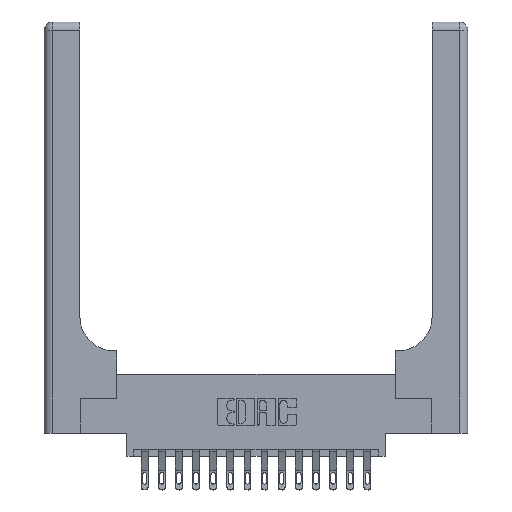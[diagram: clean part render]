
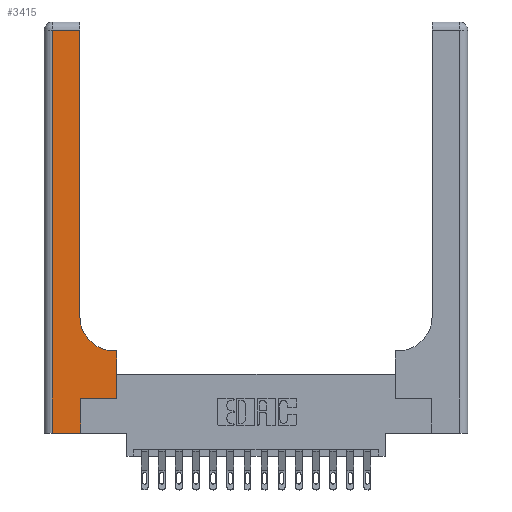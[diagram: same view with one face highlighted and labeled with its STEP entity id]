
A CAD part, top view. The second image highlights one B-rep face of the part: STEP entity #3415.
In plain terms, the highlighted planar face has unit normal (0, 0, 1).
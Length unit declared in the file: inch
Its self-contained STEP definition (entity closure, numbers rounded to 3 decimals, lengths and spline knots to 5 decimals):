
#229 = EDGE_CURVE ( 'NONE', #543, #14760, #238, .T. ) ;
#238 = LINE ( 'NONE', #16307, #10836 ) ;
#288 = VECTOR ( 'NONE', #13232, 39.37008 ) ;
#355 = ORIENTED_EDGE ( 'NONE', *, *, #1144, .T. ) ;
#386 = LINE ( 'NONE', #7572, #288 ) ;
#531 = VERTEX_POINT ( 'NONE', #16461 ) ;
#543 = VERTEX_POINT ( 'NONE', #9595 ) ;
#1144 = EDGE_CURVE ( 'NONE', #12660, #7336, #11203, .T. ) ;
#1332 = CARTESIAN_POINT ( 'NONE',  ( 0.26, 0.85, 0.37 ) ) ;
#1603 = CARTESIAN_POINT ( 'NONE',  ( 0.528, 0.25, 0.37 ) ) ;
#2816 = CARTESIAN_POINT ( 'NONE',  ( 0.265, 0.25, 0.37 ) ) ;
#2818 = EDGE_CURVE ( 'NONE', #3894, #8827, #14255, .T. ) ;
#3065 = LINE ( 'NONE', #7341, #10502 ) ;
#3185 = VERTEX_POINT ( 'NONE', #13053 ) ;
#3236 = DIRECTION ( 'NONE',  ( 0., 1., 0. ) ) ;
#3415 = ADVANCED_FACE ( 'NONE', ( #12755 ), #17022, .F. ) ;
#3499 = CARTESIAN_POINT ( 'NONE',  ( 0.51, 0.85, 0.37 ) ) ;
#3774 = CARTESIAN_POINT ( 'NONE',  ( 0.26, 2.94, 0.37 ) ) ;
#3894 = VERTEX_POINT ( 'NONE', #2816 ) ;
#3938 = VECTOR ( 'NONE', #3236, 39.37008 ) ;
#4276 = ORIENTED_EDGE ( 'NONE', *, *, #11845, .T. ) ;
#4566 = LINE ( 'NONE', #7573, #14867 ) ;
#4765 = DIRECTION ( 'NONE',  ( 0., 0., -1. ) ) ;
#5397 = EDGE_CURVE ( 'NONE', #14760, #531, #386, .T. ) ;
#5924 = ORIENTED_EDGE ( 'NONE', *, *, #5397, .T. ) ;
#5992 = AXIS2_PLACEMENT_3D ( 'NONE', #3499, #4765, #9407 ) ;
#6170 = ORIENTED_EDGE ( 'NONE', *, *, #11060, .T. ) ;
#6797 = EDGE_CURVE ( 'NONE', #7336, #9367, #3065, .T. ) ;
#6962 = CARTESIAN_POINT ( 'NONE',  ( 0.265, 0.25, 0.37 ) ) ;
#7336 = VERTEX_POINT ( 'NONE', #1332 ) ;
#7341 = CARTESIAN_POINT ( 'NONE',  ( 0.26, 3., 0.37 ) ) ;
#7572 = CARTESIAN_POINT ( 'NONE',  ( 0., 0., 0.37 ) ) ;
#7573 = CARTESIAN_POINT ( 'NONE',  ( 0., 2.94, 0.37 ) ) ;
#7842 = VECTOR ( 'NONE', #17739, 39.37008 ) ;
#8131 = ORIENTED_EDGE ( 'NONE', *, *, #11486, .T. ) ;
#8283 = DIRECTION ( 'NONE',  ( 1., 0., 0. ) ) ;
#8827 = VERTEX_POINT ( 'NONE', #18799 ) ;
#8959 = DIRECTION ( 'NONE',  ( 0., 1., 0. ) ) ;
#9367 = VERTEX_POINT ( 'NONE', #3774 ) ;
#9407 = DIRECTION ( 'NONE',  ( 1., 0., 0. ) ) ;
#9583 = DIRECTION ( 'NONE',  ( -1., 0., 0. ) ) ;
#9595 = CARTESIAN_POINT ( 'NONE',  ( 0.06, 2.94, 0.37 ) ) ;
#9724 = CARTESIAN_POINT ( 'NONE',  ( 0.06, 0., 0.37 ) ) ;
#10104 = LINE ( 'NONE', #1603, #7842 ) ;
#10468 = CARTESIAN_POINT ( 'NONE',  ( 0.265, 0., 0.37 ) ) ;
#10502 = VECTOR ( 'NONE', #8959, 39.37008 ) ;
#10836 = VECTOR ( 'NONE', #11990, 39.37008 ) ;
#11055 = DIRECTION ( 'NONE',  ( -1., 0., 0. ) ) ;
#11060 = EDGE_CURVE ( 'NONE', #9367, #543, #4566, .T. ) ;
#11203 = CIRCLE ( 'NONE', #5992, 0.25 ) ;
#11486 = EDGE_CURVE ( 'NONE', #3185, #12660, #18345, .T. ) ;
#11575 = CARTESIAN_POINT ( 'NONE',  ( 0.51, 0.6, 0.37 ) ) ;
#11688 = ORIENTED_EDGE ( 'NONE', *, *, #2818, .T. ) ;
#11845 = EDGE_CURVE ( 'NONE', #8827, #3185, #10104, .T. ) ;
#11990 = DIRECTION ( 'NONE',  ( 0., -1., 0. ) ) ;
#12189 = AXIS2_PLACEMENT_3D ( 'NONE', #13889, #18275, #9583 ) ;
#12660 = VERTEX_POINT ( 'NONE', #11575 ) ;
#12755 = FACE_OUTER_BOUND ( 'NONE', #18473, .T. ) ;
#13053 = CARTESIAN_POINT ( 'NONE',  ( 0.528, 0.6, 0.37 ) ) ;
#13232 = DIRECTION ( 'NONE',  ( 1., 0., 0. ) ) ;
#13667 = VECTOR ( 'NONE', #11055, 39.37008 ) ;
#13889 = CARTESIAN_POINT ( 'NONE',  ( 0., 3., 0.37 ) ) ;
#14255 = LINE ( 'NONE', #6962, #18006 ) ;
#14737 = ORIENTED_EDGE ( 'NONE', *, *, #6797, .T. ) ;
#14760 = VERTEX_POINT ( 'NONE', #9724 ) ;
#14867 = VECTOR ( 'NONE', #15141, 39.37008 ) ;
#15141 = DIRECTION ( 'NONE',  ( -1., 0., 0. ) ) ;
#16055 = EDGE_CURVE ( 'NONE', #531, #3894, #16316, .T. ) ;
#16307 = CARTESIAN_POINT ( 'NONE',  ( 0.06, 3., 0.37 ) ) ;
#16316 = LINE ( 'NONE', #10468, #3938 ) ;
#16461 = CARTESIAN_POINT ( 'NONE',  ( 0.265, 0., 0.37 ) ) ;
#17004 = ORIENTED_EDGE ( 'NONE', *, *, #16055, .T. ) ;
#17022 = PLANE ( 'NONE',  #12189 ) ;
#17739 = DIRECTION ( 'NONE',  ( 0., 1., 0. ) ) ;
#18006 = VECTOR ( 'NONE', #8283, 39.37008 ) ;
#18275 = DIRECTION ( 'NONE',  ( 0., 0., -1. ) ) ;
#18345 = LINE ( 'NONE', #18856, #13667 ) ;
#18473 = EDGE_LOOP ( 'NONE', ( #14737, #6170, #18868, #5924, #17004, #11688, #4276, #8131, #355 ) ) ;
#18799 = CARTESIAN_POINT ( 'NONE',  ( 0.528, 0.25, 0.37 ) ) ;
#18856 = CARTESIAN_POINT ( 'NONE',  ( 0.26, 0.6, 0.37 ) ) ;
#18868 = ORIENTED_EDGE ( 'NONE', *, *, #229, .T. ) ;
